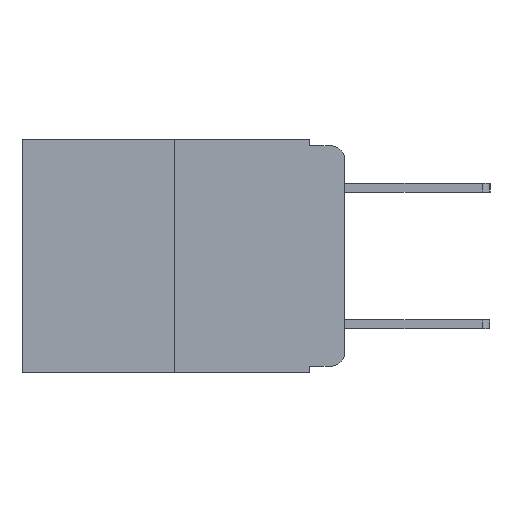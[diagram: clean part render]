
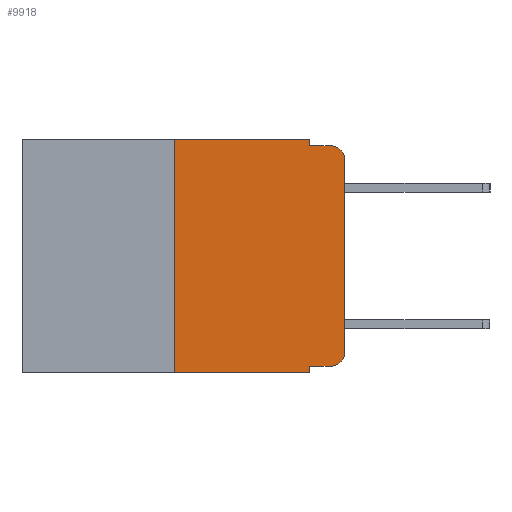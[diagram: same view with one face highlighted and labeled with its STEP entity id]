
A CAD part, left-side view. The second image highlights one B-rep face of the part: STEP entity #9918.
In plain terms, the highlighted planar face has unit normal (-1, 0, 0).
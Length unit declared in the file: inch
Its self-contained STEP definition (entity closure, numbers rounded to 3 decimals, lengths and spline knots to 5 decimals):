
#227 = CARTESIAN_POINT ( 'NONE',  ( 0., 0.051, -0.01 ) ) ;
#436 = VECTOR ( 'NONE', #6651, 39.37008 ) ;
#528 = ORIENTED_EDGE ( 'NONE', *, *, #10679, .T. ) ;
#591 = CARTESIAN_POINT ( 'NONE',  ( 0., 0.051, -0.333 ) ) ;
#703 = ORIENTED_EDGE ( 'NONE', *, *, #13397, .T. ) ;
#864 = ORIENTED_EDGE ( 'NONE', *, *, #4074, .T. ) ;
#1074 = LINE ( 'NONE', #9996, #12847 ) ;
#1216 = ORIENTED_EDGE ( 'NONE', *, *, #14595, .F. ) ;
#1229 = ORIENTED_EDGE ( 'NONE', *, *, #4787, .F. ) ;
#1416 = DIRECTION ( 'NONE',  ( 0., 0., -1. ) ) ;
#1551 = EDGE_CURVE ( 'NONE', #3567, #9522, #11261, .T. ) ;
#1611 = ORIENTED_EDGE ( 'NONE', *, *, #7160, .F. ) ;
#1693 = VECTOR ( 'NONE', #9229, 39.37008 ) ;
#1750 = DIRECTION ( 'NONE',  ( 0., -1., 0. ) ) ;
#1794 = ORIENTED_EDGE ( 'NONE', *, *, #7355, .F. ) ;
#2017 = CARTESIAN_POINT ( 'NONE',  ( 0., 0.25, -0.343 ) ) ;
#2034 = VECTOR ( 'NONE', #10346, 39.37008 ) ;
#2378 = ORIENTED_EDGE ( 'NONE', *, *, #12993, .F. ) ;
#2507 = DIRECTION ( 'NONE',  ( 0., 0., -1. ) ) ;
#2782 = ORIENTED_EDGE ( 'NONE', *, *, #13712, .T. ) ;
#2792 = ORIENTED_EDGE ( 'NONE', *, *, #1551, .T. ) ;
#2874 = LINE ( 'NONE', #591, #8334 ) ;
#3487 = CARTESIAN_POINT ( 'NONE',  ( 0., 0.02, -0.01 ) ) ;
#3567 = VERTEX_POINT ( 'NONE', #8140 ) ;
#3617 = CARTESIAN_POINT ( 'NONE',  ( 0., 0.051, -0.01 ) ) ;
#3639 = VECTOR ( 'NONE', #10143, 39.37008 ) ;
#3670 = CARTESIAN_POINT ( 'NONE',  ( 0., 0., -0.03 ) ) ;
#3756 = CARTESIAN_POINT ( 'NONE',  ( 0., 0.051, -0.333 ) ) ;
#4074 = EDGE_CURVE ( 'NONE', #8121, #12376, #13206, .T. ) ;
#4223 = AXIS2_PLACEMENT_3D ( 'NONE', #12134, #9475, #7869 ) ;
#4618 = VERTEX_POINT ( 'NONE', #12311 ) ;
#4758 = VERTEX_POINT ( 'NONE', #2017 ) ;
#4787 = EDGE_CURVE ( 'NONE', #4758, #10434, #1074, .T. ) ;
#5331 = LINE ( 'NONE', #14573, #2034 ) ;
#5851 = VERTEX_POINT ( 'NONE', #3617 ) ;
#6015 = VECTOR ( 'NONE', #1416, 39.37008 ) ;
#6651 = DIRECTION ( 'NONE',  ( 0., -1., 0. ) ) ;
#6743 = LINE ( 'NONE', #6799, #3639 ) ;
#6799 = CARTESIAN_POINT ( 'NONE',  ( 0., 0.473, -0.343 ) ) ;
#7160 = EDGE_CURVE ( 'NONE', #5851, #12376, #9615, .T. ) ;
#7355 = EDGE_CURVE ( 'NONE', #10434, #7774, #12629, .T. ) ;
#7773 = CARTESIAN_POINT ( 'NONE',  ( 0., 0.473, 0. ) ) ;
#7774 = VERTEX_POINT ( 'NONE', #13860 ) ;
#7869 = DIRECTION ( 'NONE',  ( 0., 0., -1. ) ) ;
#8121 = VERTEX_POINT ( 'NONE', #3670 ) ;
#8128 = CARTESIAN_POINT ( 'NONE',  ( 0., 0.051, 0. ) ) ;
#8140 = CARTESIAN_POINT ( 'NONE',  ( 0., 0.02, -0.333 ) ) ;
#8334 = VECTOR ( 'NONE', #1750, 39.37008 ) ;
#8639 = CARTESIAN_POINT ( 'NONE',  ( 0., 0.02, -0.03 ) ) ;
#8987 = LINE ( 'NONE', #9598, #6015 ) ;
#9229 = DIRECTION ( 'NONE',  ( 0., 0., -1. ) ) ;
#9285 = AXIS2_PLACEMENT_3D ( 'NONE', #9412, #9456, #2507 ) ;
#9412 = CARTESIAN_POINT ( 'NONE',  ( 0., 0.473, 0. ) ) ;
#9456 = DIRECTION ( 'NONE',  ( 1., 0., 0. ) ) ;
#9475 = DIRECTION ( 'NONE',  ( -1., 0., 0. ) ) ;
#9522 = VERTEX_POINT ( 'NONE', #9851 ) ;
#9598 = CARTESIAN_POINT ( 'NONE',  ( 0., 0.051, 0. ) ) ;
#9615 = LINE ( 'NONE', #227, #12142 ) ;
#9623 = DIRECTION ( 'NONE',  ( 0., -1., 0. ) ) ;
#9851 = CARTESIAN_POINT ( 'NONE',  ( 0., 0., -0.313 ) ) ;
#9918 = ADVANCED_FACE ( 'NONE', ( #10573 ), #13729, .F. ) ;
#9996 = CARTESIAN_POINT ( 'NONE',  ( 0., 0.25, 0. ) ) ;
#10143 = DIRECTION ( 'NONE',  ( 0., -1., 0. ) ) ;
#10346 = DIRECTION ( 'NONE',  ( 0., 0., 1. ) ) ;
#10434 = VERTEX_POINT ( 'NONE', #11525 ) ;
#10535 = VERTEX_POINT ( 'NONE', #3756 ) ;
#10573 = FACE_OUTER_BOUND ( 'NONE', #14351, .T. ) ;
#10679 = EDGE_CURVE ( 'NONE', #9522, #8121, #5331, .T. ) ;
#10919 = LINE ( 'NONE', #8128, #1693 ) ;
#11261 = CIRCLE ( 'NONE', #4223, 0.02 ) ;
#11525 = CARTESIAN_POINT ( 'NONE',  ( 0., 0.25, 0. ) ) ;
#12134 = CARTESIAN_POINT ( 'NONE',  ( 0., 0.02, -0.313 ) ) ;
#12142 = VECTOR ( 'NONE', #9623, 39.37008 ) ;
#12311 = CARTESIAN_POINT ( 'NONE',  ( 0., 0.051, -0.343 ) ) ;
#12376 = VERTEX_POINT ( 'NONE', #3487 ) ;
#12629 = LINE ( 'NONE', #7773, #436 ) ;
#12847 = VECTOR ( 'NONE', #14480, 39.37008 ) ;
#12993 = EDGE_CURVE ( 'NONE', #10535, #4618, #10919, .T. ) ;
#13206 = CIRCLE ( 'NONE', #14425, 0.02 ) ;
#13397 = EDGE_CURVE ( 'NONE', #10535, #3567, #2874, .T. ) ;
#13553 = DIRECTION ( 'NONE',  ( 0., 0., -1. ) ) ;
#13556 = DIRECTION ( 'NONE',  ( -1., 0., 0. ) ) ;
#13712 = EDGE_CURVE ( 'NONE', #4758, #4618, #6743, .T. ) ;
#13729 = PLANE ( 'NONE',  #9285 ) ;
#13860 = CARTESIAN_POINT ( 'NONE',  ( 0., 0.051, 0. ) ) ;
#14351 = EDGE_LOOP ( 'NONE', ( #528, #864, #1611, #1216, #1794, #1229, #2782, #2378, #703, #2792 ) ) ;
#14425 = AXIS2_PLACEMENT_3D ( 'NONE', #8639, #13556, #13553 ) ;
#14480 = DIRECTION ( 'NONE',  ( 0., 0., 1. ) ) ;
#14573 = CARTESIAN_POINT ( 'NONE',  ( 0., 0., 0. ) ) ;
#14595 = EDGE_CURVE ( 'NONE', #7774, #5851, #8987, .T. ) ;
